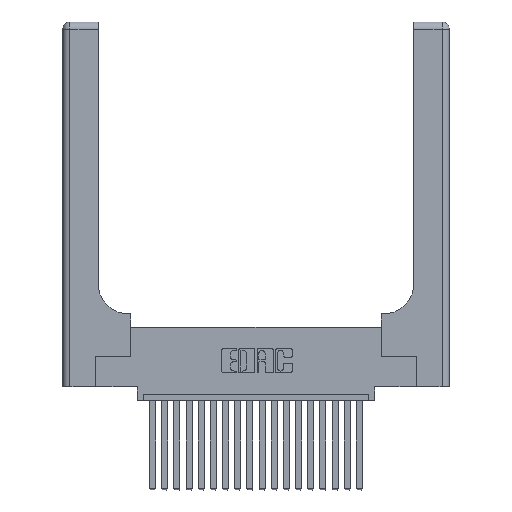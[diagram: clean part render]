
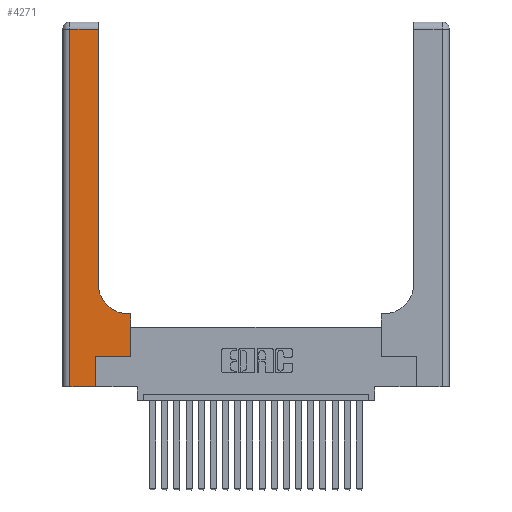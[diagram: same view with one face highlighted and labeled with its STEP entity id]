
A CAD part, top view. The second image highlights one B-rep face of the part: STEP entity #4271.
In plain terms, the highlighted planar face has unit normal (0, 0, 1).
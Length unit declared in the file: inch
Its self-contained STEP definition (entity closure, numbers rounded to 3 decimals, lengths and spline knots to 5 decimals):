
#368 = VERTEX_POINT ( 'NONE', #6474 ) ;
#1327 = CARTESIAN_POINT ( 'NONE',  ( 0.269, 0.25, 0.37 ) ) ;
#1360 = CARTESIAN_POINT ( 'NONE',  ( 0.2915, 0.6, 0.37 ) ) ;
#1651 = CARTESIAN_POINT ( 'NONE',  ( 0.5415, 0.6, 0.37 ) ) ;
#1823 = CARTESIAN_POINT ( 'NONE',  ( 0.5585, 0.25, 0.37 ) ) ;
#2595 = LINE ( 'NONE', #13410, #20092 ) ;
#2906 = AXIS2_PLACEMENT_3D ( 'NONE', #4336, #21496, #9734 ) ;
#2972 = LINE ( 'NONE', #10346, #11756 ) ;
#3114 = EDGE_LOOP ( 'NONE', ( #7040, #8811, #8076, #8431, #16149, #10350, #11604, #9348, #16995 ) ) ;
#3903 = VERTEX_POINT ( 'NONE', #10719 ) ;
#4271 = ADVANCED_FACE ( 'NONE', ( #20191 ), #18106, .F. ) ;
#4336 = CARTESIAN_POINT ( 'NONE',  ( 0., 3., 0.37 ) ) ;
#4584 = EDGE_CURVE ( 'NONE', #12165, #19489, #12747, .T. ) ;
#4952 = DIRECTION ( 'NONE',  ( 0., 1., 0. ) ) ;
#5623 = LINE ( 'NONE', #7738, #18666 ) ;
#5820 = CARTESIAN_POINT ( 'NONE',  ( 0.06, 0., 0.37 ) ) ;
#5993 = LINE ( 'NONE', #11799, #20326 ) ;
#6474 = CARTESIAN_POINT ( 'NONE',  ( 0.2915, 2.94, 0.37 ) ) ;
#7040 = ORIENTED_EDGE ( 'NONE', *, *, #21796, .T. ) ;
#7043 = EDGE_CURVE ( 'NONE', #17707, #17295, #2595, .T. ) ;
#7281 = LINE ( 'NONE', #18197, #12359 ) ;
#7738 = CARTESIAN_POINT ( 'NONE',  ( 0.269, 0., 0.37 ) ) ;
#8076 = ORIENTED_EDGE ( 'NONE', *, *, #8777, .T. ) ;
#8200 = DIRECTION ( 'NONE',  ( -1., 0., 0. ) ) ;
#8431 = ORIENTED_EDGE ( 'NONE', *, *, #8730, .T. ) ;
#8730 = EDGE_CURVE ( 'NONE', #10332, #3903, #20821, .T. ) ;
#8777 = EDGE_CURVE ( 'NONE', #10807, #10332, #7281, .T. ) ;
#8811 = ORIENTED_EDGE ( 'NONE', *, *, #9390, .T. ) ;
#9348 = ORIENTED_EDGE ( 'NONE', *, *, #4584, .T. ) ;
#9390 = EDGE_CURVE ( 'NONE', #368, #10807, #5993, .T. ) ;
#9734 = DIRECTION ( 'NONE',  ( -1., 0., 0. ) ) ;
#9937 = CARTESIAN_POINT ( 'NONE',  ( 0.2915, 0.85, 0.37 ) ) ;
#10235 = VECTOR ( 'NONE', #16014, 39.37008 ) ;
#10332 = VERTEX_POINT ( 'NONE', #5820 ) ;
#10346 = CARTESIAN_POINT ( 'NONE',  ( 0.2915, 3., 0.37 ) ) ;
#10350 = ORIENTED_EDGE ( 'NONE', *, *, #7043, .T. ) ;
#10617 = DIRECTION ( 'NONE',  ( 1., 0., 0. ) ) ;
#10719 = CARTESIAN_POINT ( 'NONE',  ( 0.269, 0., 0.37 ) ) ;
#10807 = VERTEX_POINT ( 'NONE', #13207 ) ;
#11085 = VECTOR ( 'NONE', #13728, 39.37008 ) ;
#11318 = DIRECTION ( 'NONE',  ( 0., -1., 0. ) ) ;
#11604 = ORIENTED_EDGE ( 'NONE', *, *, #18939, .T. ) ;
#11756 = VECTOR ( 'NONE', #4952, 39.37008 ) ;
#11799 = CARTESIAN_POINT ( 'NONE',  ( 0., 2.94, 0.37 ) ) ;
#12165 = VERTEX_POINT ( 'NONE', #20815 ) ;
#12359 = VECTOR ( 'NONE', #11318, 39.37008 ) ;
#12648 = DIRECTION ( 'NONE',  ( 0., 1., 0. ) ) ;
#12747 = LINE ( 'NONE', #1360, #17809 ) ;
#13207 = CARTESIAN_POINT ( 'NONE',  ( 0.06, 2.94, 0.37 ) ) ;
#13410 = CARTESIAN_POINT ( 'NONE',  ( 0.269, 0.25, 0.37 ) ) ;
#13728 = DIRECTION ( 'NONE',  ( 0., 1., 0. ) ) ;
#14393 = EDGE_CURVE ( 'NONE', #19489, #20028, #18001, .T. ) ;
#14959 = DIRECTION ( 'NONE',  ( -1., 0., 0. ) ) ;
#16014 = DIRECTION ( 'NONE',  ( 1., 0., 0. ) ) ;
#16149 = ORIENTED_EDGE ( 'NONE', *, *, #20923, .T. ) ;
#16630 = LINE ( 'NONE', #1823, #11085 ) ;
#16886 = DIRECTION ( 'NONE',  ( 1., 0., 0. ) ) ;
#16995 = ORIENTED_EDGE ( 'NONE', *, *, #14393, .T. ) ;
#17295 = VERTEX_POINT ( 'NONE', #19093 ) ;
#17707 = VERTEX_POINT ( 'NONE', #1327 ) ;
#17809 = VECTOR ( 'NONE', #14959, 39.37008 ) ;
#18001 = CIRCLE ( 'NONE', #19472, 0.25 ) ;
#18106 = PLANE ( 'NONE',  #2906 ) ;
#18197 = CARTESIAN_POINT ( 'NONE',  ( 0.06, 3., 0.37 ) ) ;
#18666 = VECTOR ( 'NONE', #12648, 39.37008 ) ;
#18939 = EDGE_CURVE ( 'NONE', #17295, #12165, #16630, .T. ) ;
#18965 = DIRECTION ( 'NONE',  ( 0., 0., -1. ) ) ;
#19093 = CARTESIAN_POINT ( 'NONE',  ( 0.5585, 0.25, 0.37 ) ) ;
#19472 = AXIS2_PLACEMENT_3D ( 'NONE', #20745, #18965, #10617 ) ;
#19489 = VERTEX_POINT ( 'NONE', #1651 ) ;
#19645 = CARTESIAN_POINT ( 'NONE',  ( 0., 0., 0.37 ) ) ;
#20028 = VERTEX_POINT ( 'NONE', #9937 ) ;
#20092 = VECTOR ( 'NONE', #16886, 39.37008 ) ;
#20191 = FACE_OUTER_BOUND ( 'NONE', #3114, .T. ) ;
#20326 = VECTOR ( 'NONE', #8200, 39.37008 ) ;
#20745 = CARTESIAN_POINT ( 'NONE',  ( 0.5415, 0.85, 0.37 ) ) ;
#20815 = CARTESIAN_POINT ( 'NONE',  ( 0.5585, 0.6, 0.37 ) ) ;
#20821 = LINE ( 'NONE', #19645, #10235 ) ;
#20923 = EDGE_CURVE ( 'NONE', #3903, #17707, #5623, .T. ) ;
#21496 = DIRECTION ( 'NONE',  ( 0., 0., -1. ) ) ;
#21796 = EDGE_CURVE ( 'NONE', #20028, #368, #2972, .T. ) ;
